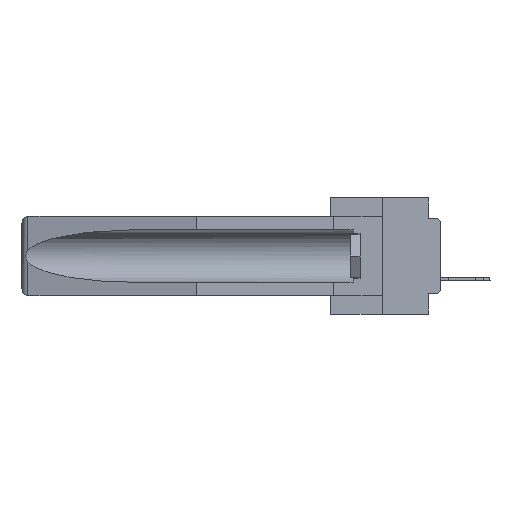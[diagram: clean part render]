
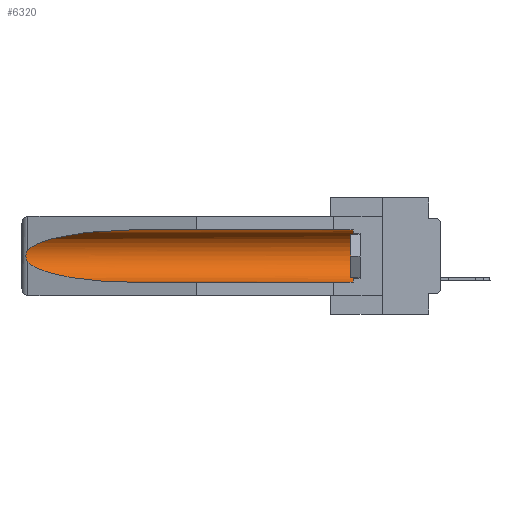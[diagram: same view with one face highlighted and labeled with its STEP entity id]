
A CAD part, left-side view. The second image highlights one B-rep face of the part: STEP entity #6320.
In plain terms, the highlighted cylindrical face has radius 2.857 mm (diameter 5.715 mm), a partial arc.
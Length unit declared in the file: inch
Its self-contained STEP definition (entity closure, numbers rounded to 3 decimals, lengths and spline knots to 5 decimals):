
#28 = VERTEX_POINT ( 'NONE', #25680 ) ;
#477 =( BOUNDED_CURVE ( )  B_SPLINE_CURVE ( 3, ( #17191, #24097, #28541, #19351 ),
 .UNSPECIFIED., .F., .F. ) 
 B_SPLINE_CURVE_WITH_KNOTS ( ( 4, 4 ),
 ( 4.71239, 6.08839 ),
 .UNSPECIFIED. ) 
 CURVE ( )  GEOMETRIC_REPRESENTATION_ITEM ( )  RATIONAL_B_SPLINE_CURVE ( ( 1., 0.848, 0.848, 1. ) ) 
 REPRESENTATION_ITEM ( '' )  );
#1034 = CARTESIAN_POINT ( 'NONE',  ( 0.26537, 1.52718, -0.14972 ) ) ;
#1181 = CARTESIAN_POINT ( 'NONE',  ( 0.26655, 1.53094, -0.18657 ) ) ;
#1525 = CARTESIAN_POINT ( 'NONE',  ( 0.155, -0.30754, -0.284 ) ) ;
#1858 = DIRECTION ( 'NONE',  ( 0., 0., 1. ) ) ;
#2029 = EDGE_LOOP ( 'NONE', ( #11774, #24727, #12398, #24318, #14897, #9639 ) ) ;
#3238 = VERTEX_POINT ( 'NONE', #3447 ) ;
#3447 = CARTESIAN_POINT ( 'NONE',  ( 0.155, 0.126, -0.059 ) ) ;
#3497 = VERTEX_POINT ( 'NONE', #20579 ) ;
#3931 = VERTEX_POINT ( 'NONE', #4126 ) ;
#4126 = CARTESIAN_POINT ( 'NONE',  ( 0.155, 0.126, -0.284 ) ) ;
#4790 = CARTESIAN_POINT ( 'NONE',  ( 0.26537, 1.52718, -0.19328 ) ) ;
#5611 =( BOUNDED_CURVE ( )  B_SPLINE_CURVE ( 3, ( #4790, #14226, #23607, #7108 ),
 .UNSPECIFIED., .F., .F. ) 
 B_SPLINE_CURVE_WITH_KNOTS ( ( 4, 4 ),
 ( 0.1948, 1.5708 ),
 .UNSPECIFIED. ) 
 CURVE ( )  GEOMETRIC_REPRESENTATION_ITEM ( )  RATIONAL_B_SPLINE_CURVE ( ( 1., 0.848, 0.848, 1. ) ) 
 REPRESENTATION_ITEM ( '' )  );
#6320 = ADVANCED_FACE ( 'NONE', ( #29572 ), #8481, .F. ) ;
#7108 = CARTESIAN_POINT ( 'NONE',  ( 0.155, 1.07973, -0.284 ) ) ;
#7818 = EDGE_CURVE ( 'NONE', #3931, #28, #12970, .T. ) ;
#8416 = CARTESIAN_POINT ( 'NONE',  ( 0.2675, 1.53308, -0.17534 ) ) ;
#8481 = CYLINDRICAL_SURFACE ( 'NONE', #23637, 0.1125 ) ;
#8491 = CARTESIAN_POINT ( 'NONE',  ( 0.155, 0.126, -0.1715 ) ) ;
#9639 = ORIENTED_EDGE ( 'NONE', *, *, #22043, .T. ) ;
#9919 = CARTESIAN_POINT ( 'NONE',  ( 0.26537, 1.52718, -0.19328 ) ) ;
#10100 = EDGE_CURVE ( 'NONE', #3497, #24780, #477, .T. ) ;
#10446 = CARTESIAN_POINT ( 'NONE',  ( 0.26654, 1.53092, -0.15636 ) ) ;
#10720 = CARTESIAN_POINT ( 'NONE',  ( 0.26537, 1.52718, -0.14972 ) ) ;
#11774 = ORIENTED_EDGE ( 'NONE', *, *, #10100, .T. ) ;
#11925 = VERTEX_POINT ( 'NONE', #9919 ) ;
#12010 = EDGE_CURVE ( 'NONE', #3931, #3238, #26774, .T. ) ;
#12289 = EDGE_CURVE ( 'NONE', #11925, #28, #5611, .T. ) ;
#12398 = ORIENTED_EDGE ( 'NONE', *, *, #12289, .T. ) ;
#12821 = DIRECTION ( 'NONE',  ( 0., 1., 0. ) ) ;
#12970 = LINE ( 'NONE', #1525, #21990 ) ;
#13553 = AXIS2_PLACEMENT_3D ( 'NONE', #8491, #17634, #27272 ) ;
#13602 = DIRECTION ( 'NONE',  ( 0., 1., 0. ) ) ;
#13759 = CARTESIAN_POINT ( 'NONE',  ( 0.155, -0.30754, -0.1715 ) ) ;
#14226 = CARTESIAN_POINT ( 'NONE',  ( 0.25451, 1.48313, -0.24835 ) ) ;
#14261 = B_SPLINE_CURVE_WITH_KNOTS ( 'NONE', 3,
 ( #1034, #22012, #10446, #24751, #26588, #8416, #19565, #1181, #19853, #20013 ),
 .UNSPECIFIED., .F., .F.,
 ( 4, 2, 2, 2, 4 ),
 ( 0., 0.00029, 0.00058, 0.00087, 0.00117 ),
 .UNSPECIFIED. ) ;
#14897 = ORIENTED_EDGE ( 'NONE', *, *, #12010, .T. ) ;
#17191 = CARTESIAN_POINT ( 'NONE',  ( 0.155, 1.07973, -0.059 ) ) ;
#17634 = DIRECTION ( 'NONE',  ( 0., -1., 0. ) ) ;
#19351 = CARTESIAN_POINT ( 'NONE',  ( 0.26537, 1.52718, -0.14972 ) ) ;
#19565 = CARTESIAN_POINT ( 'NONE',  ( 0.2673, 1.53269, -0.17917 ) ) ;
#19853 = CARTESIAN_POINT ( 'NONE',  ( 0.26597, 1.5296, -0.19026 ) ) ;
#20013 = CARTESIAN_POINT ( 'NONE',  ( 0.26537, 1.52718, -0.19328 ) ) ;
#20579 = CARTESIAN_POINT ( 'NONE',  ( 0.155, 1.07973, -0.059 ) ) ;
#21990 = VECTOR ( 'NONE', #22656, 39.37008 ) ;
#22012 = CARTESIAN_POINT ( 'NONE',  ( 0.26597, 1.52961, -0.15275 ) ) ;
#22043 = EDGE_CURVE ( 'NONE', #3238, #3497, #24488, .T. ) ;
#22653 = CARTESIAN_POINT ( 'NONE',  ( 0.155, -0.30754, -0.059 ) ) ;
#22656 = DIRECTION ( 'NONE',  ( 0., 1., 0. ) ) ;
#23607 = CARTESIAN_POINT ( 'NONE',  ( 0.21114, 1.30732, -0.284 ) ) ;
#23637 = AXIS2_PLACEMENT_3D ( 'NONE', #13759, #13602, #1858 ) ;
#24097 = CARTESIAN_POINT ( 'NONE',  ( 0.21114, 1.30732, -0.059 ) ) ;
#24318 = ORIENTED_EDGE ( 'NONE', *, *, #7818, .F. ) ;
#24488 = LINE ( 'NONE', #22653, #26956 ) ;
#24727 = ORIENTED_EDGE ( 'NONE', *, *, #29636, .T. ) ;
#24751 = CARTESIAN_POINT ( 'NONE',  ( 0.2673, 1.5327, -0.16383 ) ) ;
#24780 = VERTEX_POINT ( 'NONE', #10720 ) ;
#25680 = CARTESIAN_POINT ( 'NONE',  ( 0.155, 1.07973, -0.284 ) ) ;
#26588 = CARTESIAN_POINT ( 'NONE',  ( 0.2675, 1.53308, -0.16763 ) ) ;
#26774 = CIRCLE ( 'NONE', #13553, 0.1125 ) ;
#26956 = VECTOR ( 'NONE', #12821, 39.37008 ) ;
#27272 = DIRECTION ( 'NONE',  ( 0., 0., 1. ) ) ;
#28541 = CARTESIAN_POINT ( 'NONE',  ( 0.25451, 1.48313, -0.09465 ) ) ;
#29572 = FACE_OUTER_BOUND ( 'NONE', #2029, .T. ) ;
#29636 = EDGE_CURVE ( 'NONE', #24780, #11925, #14261, .T. ) ;
